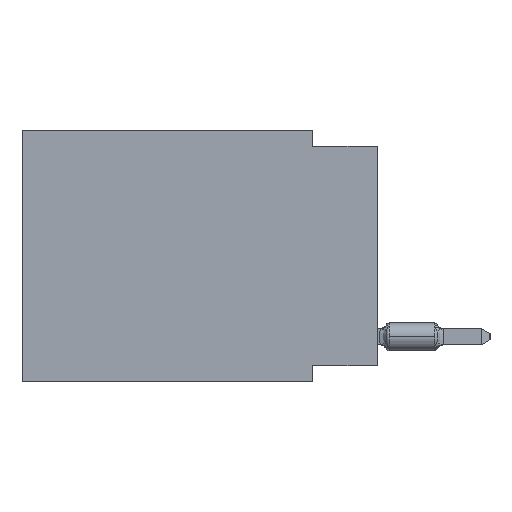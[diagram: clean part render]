
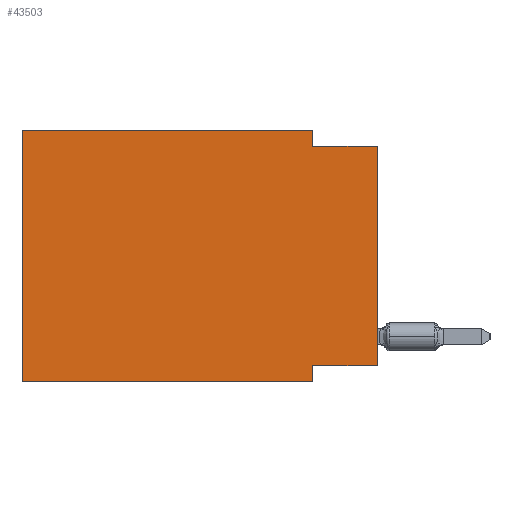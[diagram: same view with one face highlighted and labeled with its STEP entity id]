
A CAD part, left-side view. The second image highlights one B-rep face of the part: STEP entity #43503.
In plain terms, the highlighted planar face has unit normal (-1, 0, 0).
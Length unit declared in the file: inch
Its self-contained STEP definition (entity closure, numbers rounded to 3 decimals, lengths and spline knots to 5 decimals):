
#1775 = EDGE_CURVE ( 'NONE', #35771, #22606, #60923, .T. ) ;
#2268 = VERTEX_POINT ( 'NONE', #21134 ) ;
#2391 = CARTESIAN_POINT ( 'NONE',  ( 0., 0., -0.365 ) ) ;
#2535 = CARTESIAN_POINT ( 'NONE',  ( 0., 0.55, -0.39 ) ) ;
#6081 = ORIENTED_EDGE ( 'NONE', *, *, #60131, .F. ) ;
#8334 = VECTOR ( 'NONE', #65183, 39.37008 ) ;
#8856 = LINE ( 'NONE', #2391, #51198 ) ;
#9429 = DIRECTION ( 'NONE',  ( 0., -1., 0. ) ) ;
#10943 = DIRECTION ( 'NONE',  ( 0., 0., -1. ) ) ;
#11554 = EDGE_CURVE ( 'NONE', #54180, #14958, #14012, .T. ) ;
#13609 = DIRECTION ( 'NONE',  ( 0., 0., 1. ) ) ;
#14012 = LINE ( 'NONE', #32597, #21585 ) ;
#14958 = VERTEX_POINT ( 'NONE', #69288 ) ;
#16078 = AXIS2_PLACEMENT_3D ( 'NONE', #60618, #23464, #10943 ) ;
#20172 = CARTESIAN_POINT ( 'NONE',  ( 0., 0.1, -0.365 ) ) ;
#21134 = CARTESIAN_POINT ( 'NONE',  ( 0., 0.1, -0.025 ) ) ;
#21475 = CARTESIAN_POINT ( 'NONE',  ( 0., 0.1, 0. ) ) ;
#21585 = VECTOR ( 'NONE', #13609, 39.37008 ) ;
#21664 = CARTESIAN_POINT ( 'NONE',  ( 0., 0.55, 0. ) ) ;
#22038 = VERTEX_POINT ( 'NONE', #20172 ) ;
#22606 = VERTEX_POINT ( 'NONE', #49495 ) ;
#22819 = ORIENTED_EDGE ( 'NONE', *, *, #36658, .F. ) ;
#23464 = DIRECTION ( 'NONE',  ( 1., 0., 0. ) ) ;
#24348 = CARTESIAN_POINT ( 'NONE',  ( 0., 0.55, 0. ) ) ;
#25081 = VECTOR ( 'NONE', #47794, 39.37008 ) ;
#25486 = LINE ( 'NONE', #46610, #8334 ) ;
#25899 = LINE ( 'NONE', #78133, #49860 ) ;
#30581 = CARTESIAN_POINT ( 'NONE',  ( 0., 0.55, 0. ) ) ;
#30742 = ORIENTED_EDGE ( 'NONE', *, *, #34234, .F. ) ;
#32597 = CARTESIAN_POINT ( 'NONE',  ( 0., 0., 0. ) ) ;
#34234 = EDGE_CURVE ( 'NONE', #2268, #14958, #25486, .T. ) ;
#35771 = VERTEX_POINT ( 'NONE', #30581 ) ;
#36086 = EDGE_CURVE ( 'NONE', #22606, #2268, #80629, .T. ) ;
#36171 = LINE ( 'NONE', #2535, #45628 ) ;
#36658 = EDGE_CURVE ( 'NONE', #68247, #35771, #57124, .T. ) ;
#39419 = ORIENTED_EDGE ( 'NONE', *, *, #73385, .F. ) ;
#40769 = FACE_OUTER_BOUND ( 'NONE', #48704, .T. ) ;
#43503 = ADVANCED_FACE ( 'NONE', ( #40769 ), #67101, .F. ) ;
#45047 = CARTESIAN_POINT ( 'NONE',  ( 0., 0.55, -0.39 ) ) ;
#45451 = VECTOR ( 'NONE', #66159, 39.37008 ) ;
#45628 = VECTOR ( 'NONE', #9429, 39.37008 ) ;
#46610 = CARTESIAN_POINT ( 'NONE',  ( 0., 0., -0.025 ) ) ;
#47794 = DIRECTION ( 'NONE',  ( 0., 0., -1. ) ) ;
#48551 = DIRECTION ( 'NONE',  ( 0., 1., 0. ) ) ;
#48704 = EDGE_LOOP ( 'NONE', ( #65106, #30742, #48751, #55593, #22819, #53759, #6081, #39419 ) ) ;
#48751 = ORIENTED_EDGE ( 'NONE', *, *, #36086, .F. ) ;
#49495 = CARTESIAN_POINT ( 'NONE',  ( 0., 0.1, 0. ) ) ;
#49860 = VECTOR ( 'NONE', #58672, 39.37008 ) ;
#50658 = DIRECTION ( 'NONE',  ( 0., 0., 1. ) ) ;
#51198 = VECTOR ( 'NONE', #48551, 39.37008 ) ;
#53759 = ORIENTED_EDGE ( 'NONE', *, *, #59074, .T. ) ;
#54180 = VERTEX_POINT ( 'NONE', #62098 ) ;
#55593 = ORIENTED_EDGE ( 'NONE', *, *, #1775, .F. ) ;
#57124 = LINE ( 'NONE', #24348, #62354 ) ;
#58672 = DIRECTION ( 'NONE',  ( 0., 0., -1. ) ) ;
#59074 = EDGE_CURVE ( 'NONE', #68247, #73851, #36171, .T. ) ;
#60131 = EDGE_CURVE ( 'NONE', #22038, #73851, #25899, .T. ) ;
#60618 = CARTESIAN_POINT ( 'NONE',  ( 0., 0.55, 0. ) ) ;
#60923 = LINE ( 'NONE', #21664, #45451 ) ;
#62098 = CARTESIAN_POINT ( 'NONE',  ( 0., 0., -0.365 ) ) ;
#62354 = VECTOR ( 'NONE', #50658, 39.37008 ) ;
#64368 = CARTESIAN_POINT ( 'NONE',  ( 0., 0.1, -0.39 ) ) ;
#65106 = ORIENTED_EDGE ( 'NONE', *, *, #11554, .T. ) ;
#65183 = DIRECTION ( 'NONE',  ( 0., -1., 0. ) ) ;
#66159 = DIRECTION ( 'NONE',  ( 0., -1., 0. ) ) ;
#67101 = PLANE ( 'NONE',  #16078 ) ;
#68247 = VERTEX_POINT ( 'NONE', #45047 ) ;
#69288 = CARTESIAN_POINT ( 'NONE',  ( 0., 0., -0.025 ) ) ;
#73385 = EDGE_CURVE ( 'NONE', #54180, #22038, #8856, .T. ) ;
#73851 = VERTEX_POINT ( 'NONE', #64368 ) ;
#78133 = CARTESIAN_POINT ( 'NONE',  ( 0., 0.1, -0.39 ) ) ;
#80629 = LINE ( 'NONE', #21475, #25081 ) ;
